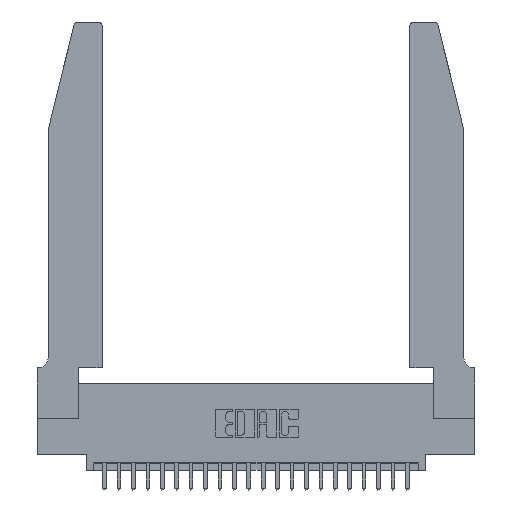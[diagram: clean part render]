
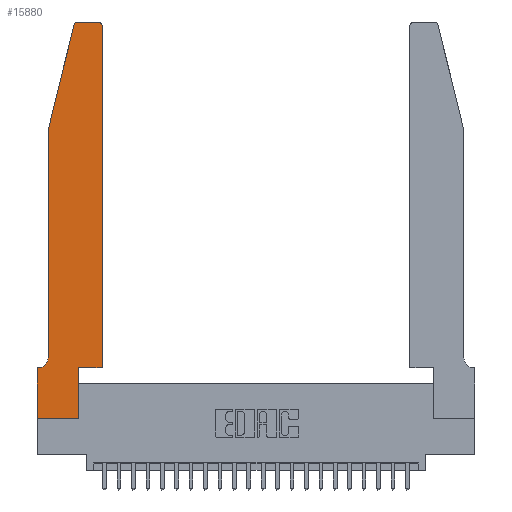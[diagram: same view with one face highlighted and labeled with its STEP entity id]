
A CAD part, top view. The second image highlights one B-rep face of the part: STEP entity #15880.
In plain terms, the highlighted planar face has unit normal (0, 0, 1).
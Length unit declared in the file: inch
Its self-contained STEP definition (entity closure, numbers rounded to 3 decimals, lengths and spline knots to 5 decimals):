
#1406 = DIRECTION ( 'NONE',  ( 1., 0., 0. ) ) ;
#1513 = LINE ( 'NONE', #19641, #11760 ) ;
#1599 = VECTOR ( 'NONE', #1406, 39.37008 ) ;
#1646 = VERTEX_POINT ( 'NONE', #5323 ) ;
#1766 = VERTEX_POINT ( 'NONE', #12473 ) ;
#2044 = DIRECTION ( 'NONE',  ( 0., 1., 0. ) ) ;
#2155 = VECTOR ( 'NONE', #9878, 39.37008 ) ;
#2697 = FACE_OUTER_BOUND ( 'NONE', #18546, .T. ) ;
#2715 = EDGE_CURVE ( 'NONE', #4693, #1766, #21227, .T. ) ;
#2976 = ORIENTED_EDGE ( 'NONE', *, *, #11734, .T. ) ;
#3039 = ORIENTED_EDGE ( 'NONE', *, *, #20170, .T. ) ;
#3085 = CARTESIAN_POINT ( 'NONE',  ( 0., 0.35, 0.37 ) ) ;
#3121 = CARTESIAN_POINT ( 'NONE',  ( 0.0755, 0.42, 0.37 ) ) ;
#3155 = AXIS2_PLACEMENT_3D ( 'NONE', #10230, #23578, #12139 ) ;
#3199 = EDGE_CURVE ( 'NONE', #10809, #14328, #21203, .T. ) ;
#3948 = CARTESIAN_POINT ( 'NONE',  ( 0., 0., 0.37 ) ) ;
#4693 = VERTEX_POINT ( 'NONE', #20967 ) ;
#5009 = DIRECTION ( 'NONE',  ( 1., 0., 0. ) ) ;
#5074 = ORIENTED_EDGE ( 'NONE', *, *, #21087, .T. ) ;
#5086 = DIRECTION ( 'NONE',  ( -1., 0., 0. ) ) ;
#5100 = VERTEX_POINT ( 'NONE', #22088 ) ;
#5323 = CARTESIAN_POINT ( 'NONE',  ( 0.2865, 0., 0.37 ) ) ;
#5541 = ORIENTED_EDGE ( 'NONE', *, *, #8643, .T. ) ;
#5628 = LINE ( 'NONE', #19847, #10766 ) ;
#5694 = CIRCLE ( 'NONE', #3155, 0.03 ) ;
#5859 = VECTOR ( 'NONE', #2044, 39.37008 ) ;
#5867 = DIRECTION ( 'NONE',  ( 0., -1., 0. ) ) ;
#6198 = EDGE_CURVE ( 'NONE', #14328, #19764, #17783, .T. ) ;
#6734 = LINE ( 'NONE', #18527, #1599 ) ;
#7312 = LINE ( 'NONE', #19395, #2155 ) ;
#7476 = EDGE_CURVE ( 'NONE', #11594, #4693, #1513, .T. ) ;
#7746 = VERTEX_POINT ( 'NONE', #3121 ) ;
#8042 = DIRECTION ( 'NONE',  ( 0., 0., -1. ) ) ;
#8164 = AXIS2_PLACEMENT_3D ( 'NONE', #22951, #11513, #24873 ) ;
#8643 = EDGE_CURVE ( 'NONE', #7746, #10809, #21677, .T. ) ;
#8674 = CARTESIAN_POINT ( 'NONE',  ( 0.4205, 2.75, 0.37 ) ) ;
#8958 = CARTESIAN_POINT ( 'NONE',  ( 0., 0., 0.37 ) ) ;
#9878 = DIRECTION ( 'NONE',  ( -1., 0., 0. ) ) ;
#10015 = ORIENTED_EDGE ( 'NONE', *, *, #3199, .T. ) ;
#10038 = DIRECTION ( 'NONE',  ( 1., 0., 0. ) ) ;
#10230 = CARTESIAN_POINT ( 'NONE',  ( 0.4205, 2.72, 0.37 ) ) ;
#10468 = VECTOR ( 'NONE', #13398, 39.37008 ) ;
#10719 = ORIENTED_EDGE ( 'NONE', *, *, #6198, .T. ) ;
#10766 = VECTOR ( 'NONE', #15990, 39.37008 ) ;
#10809 = VERTEX_POINT ( 'NONE', #12699 ) ;
#10884 = CARTESIAN_POINT ( 'NONE',  ( 0.0755, 2., 0.37 ) ) ;
#10998 = ORIENTED_EDGE ( 'NONE', *, *, #7476, .T. ) ;
#11018 = ORIENTED_EDGE ( 'NONE', *, *, #2715, .T. ) ;
#11513 = DIRECTION ( 'NONE',  ( 0., 0., 1. ) ) ;
#11594 = VERTEX_POINT ( 'NONE', #17818 ) ;
#11734 = EDGE_CURVE ( 'NONE', #1766, #24699, #5694, .T. ) ;
#11760 = VECTOR ( 'NONE', #10038, 39.37008 ) ;
#11892 = CARTESIAN_POINT ( 'NONE',  ( 0.4505, 0.35, 0.37 ) ) ;
#12139 = DIRECTION ( 'NONE',  ( 1., 0., 0. ) ) ;
#12473 = CARTESIAN_POINT ( 'NONE',  ( 0.4505, 2.72, 0.37 ) ) ;
#12699 = CARTESIAN_POINT ( 'NONE',  ( 0.0055, 0.35, 0.37 ) ) ;
#12760 = EDGE_CURVE ( 'NONE', #12786, #5100, #20021, .T. ) ;
#12786 = VERTEX_POINT ( 'NONE', #13451 ) ;
#13398 = DIRECTION ( 'NONE',  ( 0., 1., 0. ) ) ;
#13451 = CARTESIAN_POINT ( 'NONE',  ( 0.284, 2.75, 0.37 ) ) ;
#13587 = CARTESIAN_POINT ( 'NONE',  ( 0.2865, 0.35, 0.37 ) ) ;
#14328 = VERTEX_POINT ( 'NONE', #22210 ) ;
#14684 = CARTESIAN_POINT ( 'NONE',  ( 0.0755, 0.35, 0.37 ) ) ;
#15497 = VECTOR ( 'NONE', #5086, 39.37008 ) ;
#15616 = CARTESIAN_POINT ( 'NONE',  ( 0.0755, 2., 0.37 ) ) ;
#15880 = ADVANCED_FACE ( 'NONE', ( #2697 ), #16437, .T. ) ;
#15990 = DIRECTION ( 'NONE',  ( 0., -1., 0. ) ) ;
#16437 = PLANE ( 'NONE',  #16710 ) ;
#16518 = DIRECTION ( 'NONE',  ( 0., 0., 1. ) ) ;
#16710 = AXIS2_PLACEMENT_3D ( 'NONE', #3085, #16518, #5009 ) ;
#16965 = ORIENTED_EDGE ( 'NONE', *, *, #19511, .T. ) ;
#17475 = LINE ( 'NONE', #15616, #21954 ) ;
#17783 = LINE ( 'NONE', #3948, #22868 ) ;
#17818 = CARTESIAN_POINT ( 'NONE',  ( 0.2865, 0.35, 0.37 ) ) ;
#18218 = ORIENTED_EDGE ( 'NONE', *, *, #21652, .T. ) ;
#18527 = CARTESIAN_POINT ( 'NONE',  ( 0., 0., 0.37 ) ) ;
#18546 = EDGE_LOOP ( 'NONE', ( #5074, #22202, #22252, #18218, #5541, #10015, #10719, #3039, #16965, #10998, #11018, #2976 ) ) ;
#19395 = CARTESIAN_POINT ( 'NONE',  ( 0.2605, 2.75, 0.37 ) ) ;
#19474 = DIRECTION ( 'NONE',  ( -0.239, -0.971, 0. ) ) ;
#19503 = CARTESIAN_POINT ( 'NONE',  ( 0.0055, 0.42, 0.37 ) ) ;
#19511 = EDGE_CURVE ( 'NONE', #1646, #11594, #21163, .T. ) ;
#19641 = CARTESIAN_POINT ( 'NONE',  ( 0.4505, 0.35, 0.37 ) ) ;
#19764 = VERTEX_POINT ( 'NONE', #8958 ) ;
#19847 = CARTESIAN_POINT ( 'NONE',  ( 0.0755, 2., 0.37 ) ) ;
#20021 = CIRCLE ( 'NONE', #8164, 0.03 ) ;
#20170 = EDGE_CURVE ( 'NONE', #19764, #1646, #6734, .T. ) ;
#20798 = AXIS2_PLACEMENT_3D ( 'NONE', #19503, #8042, #21412 ) ;
#20967 = CARTESIAN_POINT ( 'NONE',  ( 0.4505, 0.35, 0.37 ) ) ;
#21087 = EDGE_CURVE ( 'NONE', #24699, #12786, #7312, .T. ) ;
#21127 = EDGE_CURVE ( 'NONE', #5100, #22542, #17475, .T. ) ;
#21163 = LINE ( 'NONE', #13587, #5859 ) ;
#21203 = LINE ( 'NONE', #14684, #15497 ) ;
#21227 = LINE ( 'NONE', #11892, #10468 ) ;
#21412 = DIRECTION ( 'NONE',  ( -1., 0., 0. ) ) ;
#21652 = EDGE_CURVE ( 'NONE', #22542, #7746, #5628, .T. ) ;
#21677 = CIRCLE ( 'NONE', #20798, 0.07 ) ;
#21954 = VECTOR ( 'NONE', #19474, 39.37008 ) ;
#22088 = CARTESIAN_POINT ( 'NONE',  ( 0.25487, 2.72718, 0.37 ) ) ;
#22202 = ORIENTED_EDGE ( 'NONE', *, *, #12760, .T. ) ;
#22210 = CARTESIAN_POINT ( 'NONE',  ( 0., 0.35, 0.37 ) ) ;
#22252 = ORIENTED_EDGE ( 'NONE', *, *, #21127, .T. ) ;
#22542 = VERTEX_POINT ( 'NONE', #10884 ) ;
#22868 = VECTOR ( 'NONE', #5867, 39.37008 ) ;
#22951 = CARTESIAN_POINT ( 'NONE',  ( 0.284, 2.72, 0.37 ) ) ;
#23578 = DIRECTION ( 'NONE',  ( 0., 0., 1. ) ) ;
#24699 = VERTEX_POINT ( 'NONE', #8674 ) ;
#24873 = DIRECTION ( 'NONE',  ( 1., 0., 0. ) ) ;
